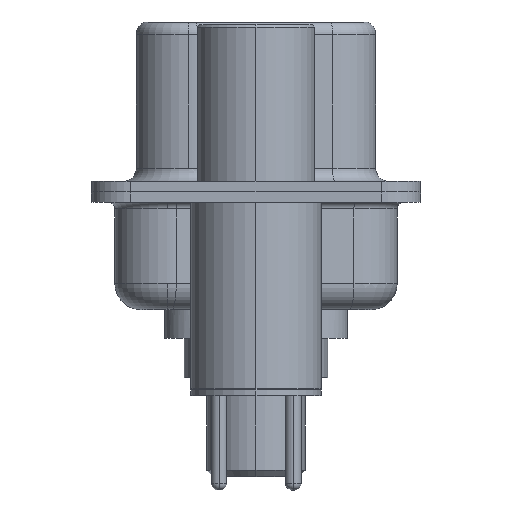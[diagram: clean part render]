
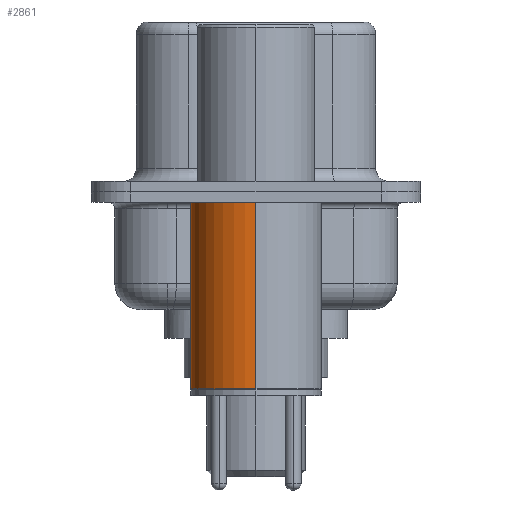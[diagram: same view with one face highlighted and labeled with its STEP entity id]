
A CAD part, left-side view. The second image highlights one B-rep face of the part: STEP entity #2861.
In plain terms, the highlighted cylindrical face has radius 2.5 mm (diameter 5 mm), a partial arc.
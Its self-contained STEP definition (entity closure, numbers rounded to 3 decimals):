
#812 = VECTOR ( 'NONE', #17179, 1000. ) ;
#1100 = CARTESIAN_POINT ( 'NONE',  ( 0., 0., -7.525 ) ) ;
#2509 = CARTESIAN_POINT ( 'NONE',  ( -2.5, 0., -7.525 ) ) ;
#2570 = DIRECTION ( 'NONE',  ( 1., 0., 0. ) ) ;
#2861 = ADVANCED_FACE ( 'NONE', ( #4400 ), #11717, .T. ) ;
#3121 = ORIENTED_EDGE ( 'NONE', *, *, #16740, .T. ) ;
#3355 = VERTEX_POINT ( 'NONE', #10375 ) ;
#3511 = CARTESIAN_POINT ( 'NONE',  ( 0., 0., 0.581 ) ) ;
#4150 = ORIENTED_EDGE ( 'NONE', *, *, #15079, .T. ) ;
#4400 = FACE_OUTER_BOUND ( 'NONE', #9395, .T. ) ;
#4706 = LINE ( 'NONE', #15811, #812 ) ;
#6149 = CARTESIAN_POINT ( 'NONE',  ( 0., 0., -0.4 ) ) ;
#6524 = EDGE_CURVE ( 'NONE', #7468, #3355, #18182, .T. ) ;
#6778 = VECTOR ( 'NONE', #13153, 1000. ) ;
#7334 = CARTESIAN_POINT ( 'NONE',  ( -2.5, 0., 0.581 ) ) ;
#7445 = DIRECTION ( 'NONE',  ( 1., 0., 0. ) ) ;
#7468 = VERTEX_POINT ( 'NONE', #8084 ) ;
#7621 = DIRECTION ( 'NONE',  ( 1., 0., 0. ) ) ;
#8084 = CARTESIAN_POINT ( 'NONE',  ( 2.5, 0., -0.4 ) ) ;
#8187 = VERTEX_POINT ( 'NONE', #2509 ) ;
#8865 = CARTESIAN_POINT ( 'NONE',  ( 2.5, 0., -7.525 ) ) ;
#9395 = EDGE_LOOP ( 'NONE', ( #3121, #4150, #10202, #14175 ) ) ;
#10202 = ORIENTED_EDGE ( 'NONE', *, *, #6524, .F. ) ;
#10375 = CARTESIAN_POINT ( 'NONE',  ( -2.5, 0., -0.4 ) ) ;
#10577 = AXIS2_PLACEMENT_3D ( 'NONE', #3511, #13553, #7445 ) ;
#11271 = DIRECTION ( 'NONE',  ( 0., 0., 1. ) ) ;
#11717 = CYLINDRICAL_SURFACE ( 'NONE', #10577, 2.5 ) ;
#13122 = AXIS2_PLACEMENT_3D ( 'NONE', #1100, #11271, #2570 ) ;
#13153 = DIRECTION ( 'NONE',  ( 0., 0., 1. ) ) ;
#13553 = DIRECTION ( 'NONE',  ( 0., 0., 1. ) ) ;
#13628 = AXIS2_PLACEMENT_3D ( 'NONE', #6149, #16337, #7621 ) ;
#14175 = ORIENTED_EDGE ( 'NONE', *, *, #14971, .F. ) ;
#14548 = LINE ( 'NONE', #7334, #6778 ) ;
#14674 = VERTEX_POINT ( 'NONE', #8865 ) ;
#14971 = EDGE_CURVE ( 'NONE', #14674, #7468, #4706, .T. ) ;
#15079 = EDGE_CURVE ( 'NONE', #8187, #3355, #14548, .T. ) ;
#15811 = CARTESIAN_POINT ( 'NONE',  ( 2.5, 0., 0.581 ) ) ;
#16337 = DIRECTION ( 'NONE',  ( 0., 0., 1. ) ) ;
#16740 = EDGE_CURVE ( 'NONE', #14674, #8187, #17650, .T. ) ;
#17179 = DIRECTION ( 'NONE',  ( 0., 0., 1. ) ) ;
#17650 = CIRCLE ( 'NONE', #13122, 2.5 ) ;
#18182 = CIRCLE ( 'NONE', #13628, 2.5 ) ;
